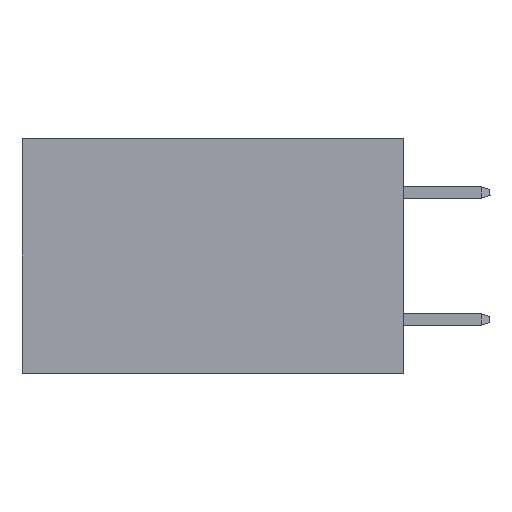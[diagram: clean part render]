
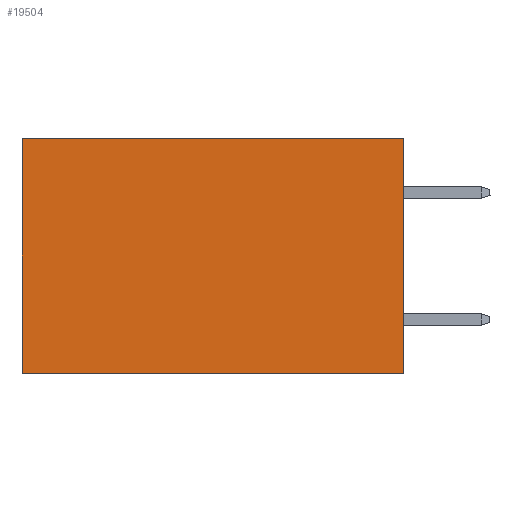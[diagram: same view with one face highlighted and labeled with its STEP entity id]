
A CAD part, left-side view. The second image highlights one B-rep face of the part: STEP entity #19504.
In plain terms, the highlighted planar face has unit normal (-1, 0, 0).
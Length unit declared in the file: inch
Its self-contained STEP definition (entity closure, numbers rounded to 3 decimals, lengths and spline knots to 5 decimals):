
#1193 = ORIENTED_EDGE ( 'NONE', *, *, #18621, .T. ) ;
#1983 = CARTESIAN_POINT ( 'NONE',  ( 0.2875, 0., -0.37 ) ) ;
#2115 = VECTOR ( 'NONE', #23563, 39.37008 ) ;
#2594 = DIRECTION ( 'NONE',  ( 0., 0., -1. ) ) ;
#2675 = EDGE_LOOP ( 'NONE', ( #1193, #18493, #23321, #3983 ) ) ;
#2943 = DIRECTION ( 'NONE',  ( 0., 1., 0. ) ) ;
#3053 = CARTESIAN_POINT ( 'NONE',  ( 0.2875, 0., 0. ) ) ;
#3087 = LINE ( 'NONE', #22154, #21036 ) ;
#3664 = VECTOR ( 'NONE', #18693, 39.37008 ) ;
#3983 = ORIENTED_EDGE ( 'NONE', *, *, #9692, .T. ) ;
#4220 = CARTESIAN_POINT ( 'NONE',  ( 0.2875, 0.6, 0. ) ) ;
#4760 = DIRECTION ( 'NONE',  ( 0., 0., -1. ) ) ;
#5434 = VERTEX_POINT ( 'NONE', #19653 ) ;
#5856 = VECTOR ( 'NONE', #4760, 39.37008 ) ;
#6656 = EDGE_CURVE ( 'NONE', #5434, #11202, #18731, .T. ) ;
#7574 = PLANE ( 'NONE',  #12861 ) ;
#9692 = EDGE_CURVE ( 'NONE', #5434, #29790, #3087, .T. ) ;
#9940 = FACE_OUTER_BOUND ( 'NONE', #2675, .T. ) ;
#11202 = VERTEX_POINT ( 'NONE', #29366 ) ;
#12071 = CARTESIAN_POINT ( 'NONE',  ( 0.2875, 0.6, 0. ) ) ;
#12861 = AXIS2_PLACEMENT_3D ( 'NONE', #3053, #21663, #2594 ) ;
#16395 = CARTESIAN_POINT ( 'NONE',  ( 0.2875, 0., 0. ) ) ;
#17172 = VERTEX_POINT ( 'NONE', #18914 ) ;
#18493 = ORIENTED_EDGE ( 'NONE', *, *, #30236, .F. ) ;
#18621 = EDGE_CURVE ( 'NONE', #29790, #17172, #23948, .T. ) ;
#18693 = DIRECTION ( 'NONE',  ( 0., 1., 0. ) ) ;
#18731 = LINE ( 'NONE', #16395, #2115 ) ;
#18914 = CARTESIAN_POINT ( 'NONE',  ( 0.2875, 0.6, -0.37 ) ) ;
#19504 = ADVANCED_FACE ( 'NONE', ( #9940 ), #7574, .F. ) ;
#19653 = CARTESIAN_POINT ( 'NONE',  ( 0.2875, 0., 0. ) ) ;
#21036 = VECTOR ( 'NONE', #2943, 39.37008 ) ;
#21663 = DIRECTION ( 'NONE',  ( 1., 0., 0. ) ) ;
#22154 = CARTESIAN_POINT ( 'NONE',  ( 0.2875, 0., 0. ) ) ;
#23321 = ORIENTED_EDGE ( 'NONE', *, *, #6656, .F. ) ;
#23563 = DIRECTION ( 'NONE',  ( 0., 0., -1. ) ) ;
#23948 = LINE ( 'NONE', #12071, #5856 ) ;
#25714 = LINE ( 'NONE', #1983, #3664 ) ;
#29366 = CARTESIAN_POINT ( 'NONE',  ( 0.2875, 0., -0.37 ) ) ;
#29790 = VERTEX_POINT ( 'NONE', #4220 ) ;
#30236 = EDGE_CURVE ( 'NONE', #11202, #17172, #25714, .T. ) ;
